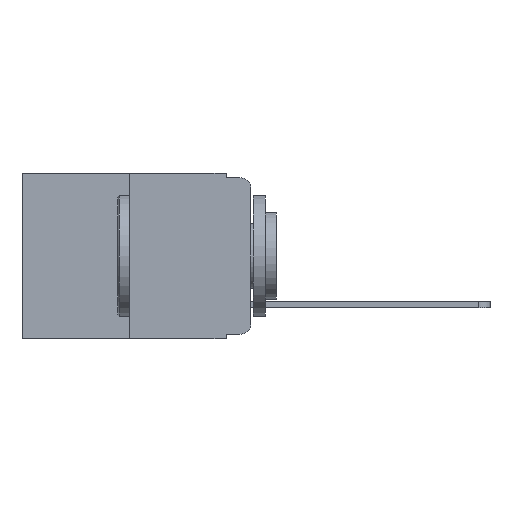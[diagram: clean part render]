
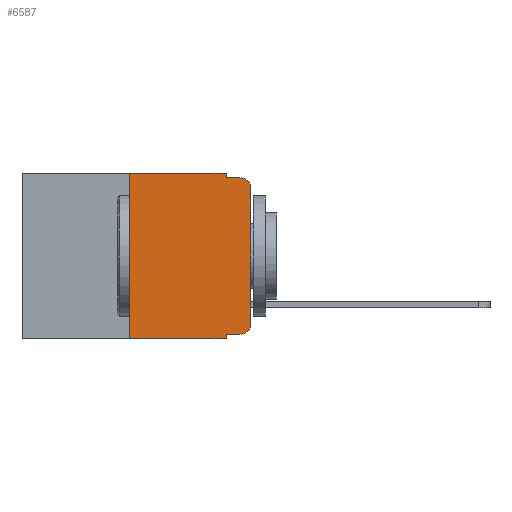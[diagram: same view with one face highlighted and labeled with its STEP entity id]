
A CAD part, left-side view. The second image highlights one B-rep face of the part: STEP entity #6587.
In plain terms, the highlighted planar face has unit normal (-1, 0, 0).
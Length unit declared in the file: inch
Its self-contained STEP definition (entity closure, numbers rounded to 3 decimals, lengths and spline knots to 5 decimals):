
#123 = CARTESIAN_POINT ( 'NONE',  ( 0., 0.051, -0.333 ) ) ;
#291 = ORIENTED_EDGE ( 'NONE', *, *, #9450, .T. ) ;
#394 = LINE ( 'NONE', #1651, #9092 ) ;
#577 = EDGE_CURVE ( 'NONE', #5483, #14189, #4067, .T. ) ;
#600 = EDGE_CURVE ( 'NONE', #12531, #10465, #5169, .T. ) ;
#826 = LINE ( 'NONE', #6866, #11002 ) ;
#1024 = CARTESIAN_POINT ( 'NONE',  ( 0., 0.473, -0.343 ) ) ;
#1391 = CARTESIAN_POINT ( 'NONE',  ( 0., 0.25, 0. ) ) ;
#1564 = CARTESIAN_POINT ( 'NONE',  ( 0., 0.473, 0. ) ) ;
#1565 = LINE ( 'NONE', #3067, #13577 ) ;
#1651 = CARTESIAN_POINT ( 'NONE',  ( 0., 0.051, -0.01 ) ) ;
#2117 = DIRECTION ( 'NONE',  ( 0., 0., -1. ) ) ;
#2124 = DIRECTION ( 'NONE',  ( 0., -1., 0. ) ) ;
#2385 = EDGE_CURVE ( 'NONE', #12962, #13815, #394, .T. ) ;
#2640 = ORIENTED_EDGE ( 'NONE', *, *, #2385, .F. ) ;
#2721 = EDGE_LOOP ( 'NONE', ( #291, #12108, #2640, #12033, #2758, #8648, #13820, #14600, #13639, #6488 ) ) ;
#2758 = ORIENTED_EDGE ( 'NONE', *, *, #600, .F. ) ;
#2890 = DIRECTION ( 'NONE',  ( -1., 0., 0. ) ) ;
#3067 = CARTESIAN_POINT ( 'NONE',  ( 0., 0.051, 0. ) ) ;
#3120 = CARTESIAN_POINT ( 'NONE',  ( 0., 0.02, -0.333 ) ) ;
#3610 = CIRCLE ( 'NONE', #9539, 0.02 ) ;
#3750 = DIRECTION ( 'NONE',  ( 0., -1., 0. ) ) ;
#3848 = AXIS2_PLACEMENT_3D ( 'NONE', #14280, #13148, #3903 ) ;
#3903 = DIRECTION ( 'NONE',  ( 0., 0., -1. ) ) ;
#3982 = AXIS2_PLACEMENT_3D ( 'NONE', #8463, #9616, #14326 ) ;
#4054 = DIRECTION ( 'NONE',  ( 0., 0., -1. ) ) ;
#4067 = CIRCLE ( 'NONE', #3982, 0.02 ) ;
#4069 = CARTESIAN_POINT ( 'NONE',  ( 0., 0.02, -0.01 ) ) ;
#5075 = EDGE_CURVE ( 'NONE', #10129, #8633, #6850, .T. ) ;
#5145 = EDGE_CURVE ( 'NONE', #11142, #5483, #9191, .T. ) ;
#5169 = LINE ( 'NONE', #1564, #10972 ) ;
#5214 = VECTOR ( 'NONE', #14900, 39.37008 ) ;
#5483 = VERTEX_POINT ( 'NONE', #3120 ) ;
#5489 = EDGE_CURVE ( 'NONE', #10465, #12962, #1565, .T. ) ;
#5702 = EDGE_CURVE ( 'NONE', #11142, #8633, #826, .T. ) ;
#6124 = VERTEX_POINT ( 'NONE', #14778 ) ;
#6150 = CARTESIAN_POINT ( 'NONE',  ( 0., 0., -0.313 ) ) ;
#6488 = ORIENTED_EDGE ( 'NONE', *, *, #577, .T. ) ;
#6587 = ADVANCED_FACE ( 'NONE', ( #7137 ), #13245, .F. ) ;
#6790 = CARTESIAN_POINT ( 'NONE',  ( 0., 0.051, -0.333 ) ) ;
#6850 = LINE ( 'NONE', #1024, #11370 ) ;
#6866 = CARTESIAN_POINT ( 'NONE',  ( 0., 0.051, 0. ) ) ;
#7137 = FACE_OUTER_BOUND ( 'NONE', #2721, .T. ) ;
#7576 = CARTESIAN_POINT ( 'NONE',  ( 0., 0.25, -0.343 ) ) ;
#7963 = CARTESIAN_POINT ( 'NONE',  ( 0., 0.051, -0.01 ) ) ;
#8463 = CARTESIAN_POINT ( 'NONE',  ( 0., 0.02, -0.313 ) ) ;
#8633 = VERTEX_POINT ( 'NONE', #13812 ) ;
#8648 = ORIENTED_EDGE ( 'NONE', *, *, #11866, .F. ) ;
#9092 = VECTOR ( 'NONE', #10990, 39.37008 ) ;
#9191 = LINE ( 'NONE', #6790, #5214 ) ;
#9450 = EDGE_CURVE ( 'NONE', #14189, #6124, #14211, .T. ) ;
#9539 = AXIS2_PLACEMENT_3D ( 'NONE', #9821, #2890, #4054 ) ;
#9616 = DIRECTION ( 'NONE',  ( -1., 0., 0. ) ) ;
#9621 = DIRECTION ( 'NONE',  ( 0., 0., 1. ) ) ;
#9821 = CARTESIAN_POINT ( 'NONE',  ( 0., 0.02, -0.03 ) ) ;
#10097 = DIRECTION ( 'NONE',  ( 0., 0., -1. ) ) ;
#10129 = VERTEX_POINT ( 'NONE', #7576 ) ;
#10465 = VERTEX_POINT ( 'NONE', #14951 ) ;
#10579 = LINE ( 'NONE', #1391, #10931 ) ;
#10931 = VECTOR ( 'NONE', #14122, 39.37008 ) ;
#10972 = VECTOR ( 'NONE', #3750, 39.37008 ) ;
#10990 = DIRECTION ( 'NONE',  ( 0., -1., 0. ) ) ;
#11002 = VECTOR ( 'NONE', #2117, 39.37008 ) ;
#11142 = VERTEX_POINT ( 'NONE', #123 ) ;
#11370 = VECTOR ( 'NONE', #2124, 39.37008 ) ;
#11518 = EDGE_CURVE ( 'NONE', #6124, #13815, #3610, .T. ) ;
#11866 = EDGE_CURVE ( 'NONE', #10129, #12531, #10579, .T. ) ;
#12033 = ORIENTED_EDGE ( 'NONE', *, *, #5489, .F. ) ;
#12108 = ORIENTED_EDGE ( 'NONE', *, *, #11518, .T. ) ;
#12531 = VERTEX_POINT ( 'NONE', #12966 ) ;
#12962 = VERTEX_POINT ( 'NONE', #7963 ) ;
#12966 = CARTESIAN_POINT ( 'NONE',  ( 0., 0.25, 0. ) ) ;
#13148 = DIRECTION ( 'NONE',  ( 1., 0., 0. ) ) ;
#13245 = PLANE ( 'NONE',  #3848 ) ;
#13577 = VECTOR ( 'NONE', #10097, 39.37008 ) ;
#13639 = ORIENTED_EDGE ( 'NONE', *, *, #5145, .T. ) ;
#13812 = CARTESIAN_POINT ( 'NONE',  ( 0., 0.051, -0.343 ) ) ;
#13815 = VERTEX_POINT ( 'NONE', #4069 ) ;
#13820 = ORIENTED_EDGE ( 'NONE', *, *, #5075, .T. ) ;
#13834 = VECTOR ( 'NONE', #9621, 39.37008 ) ;
#14122 = DIRECTION ( 'NONE',  ( 0., 0., 1. ) ) ;
#14189 = VERTEX_POINT ( 'NONE', #6150 ) ;
#14211 = LINE ( 'NONE', #14246, #13834 ) ;
#14246 = CARTESIAN_POINT ( 'NONE',  ( 0., 0., 0. ) ) ;
#14280 = CARTESIAN_POINT ( 'NONE',  ( 0., 0.473, 0. ) ) ;
#14326 = DIRECTION ( 'NONE',  ( 0., 0., -1. ) ) ;
#14600 = ORIENTED_EDGE ( 'NONE', *, *, #5702, .F. ) ;
#14778 = CARTESIAN_POINT ( 'NONE',  ( 0., 0., -0.03 ) ) ;
#14900 = DIRECTION ( 'NONE',  ( 0., -1., 0. ) ) ;
#14951 = CARTESIAN_POINT ( 'NONE',  ( 0., 0.051, 0. ) ) ;
